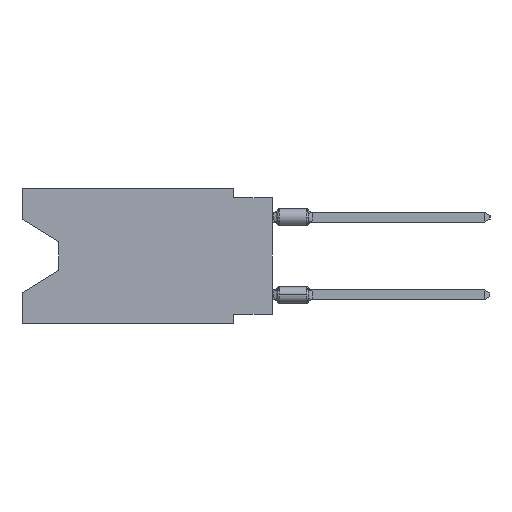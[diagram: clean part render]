
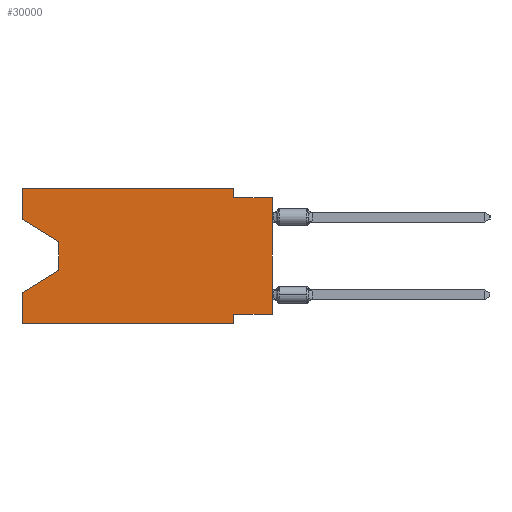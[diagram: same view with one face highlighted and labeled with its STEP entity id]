
A CAD part, left-side view. The second image highlights one B-rep face of the part: STEP entity #30000.
In plain terms, the highlighted planar face has unit normal (-1, 0, 0).
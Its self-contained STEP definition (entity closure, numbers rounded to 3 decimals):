
#176 = ORIENTED_EDGE ( 'NONE', *, *, #2564, .F. ) ;
#928 = VECTOR ( 'NONE', #32662, 1000. ) ;
#1116 = EDGE_CURVE ( 'NONE', #18634, #1347, #31646, .T. ) ;
#1347 = VERTEX_POINT ( 'NONE', #36862 ) ;
#2201 = DIRECTION ( 'NONE',  ( 0., 0., -1. ) ) ;
#2564 = EDGE_CURVE ( 'NONE', #3767, #1347, #11342, .T. ) ;
#3525 = VERTEX_POINT ( 'NONE', #20771 ) ;
#3580 = DIRECTION ( 'NONE',  ( 0., 0., 1. ) ) ;
#3767 = VERTEX_POINT ( 'NONE', #25257 ) ;
#4405 = EDGE_CURVE ( 'NONE', #15821, #12449, #11869, .T. ) ;
#4849 = CARTESIAN_POINT ( 'NONE',  ( 0., 13.97, -5.385 ) ) ;
#4953 = VECTOR ( 'NONE', #6127, 1000. ) ;
#4959 = DIRECTION ( 'NONE',  ( 0., -1., 0. ) ) ;
#5584 = CARTESIAN_POINT ( 'NONE',  ( 0., 2.54, -8.89 ) ) ;
#6069 = ORIENTED_EDGE ( 'NONE', *, *, #1116, .T. ) ;
#6127 = DIRECTION ( 'NONE',  ( 0., 1., 0. ) ) ;
#7717 = LINE ( 'NONE', #35167, #36798 ) ;
#8383 = DIRECTION ( 'NONE',  ( 0., -1., 0. ) ) ;
#9143 = CARTESIAN_POINT ( 'NONE',  ( 0., 13.97, -3.505 ) ) ;
#9159 = EDGE_CURVE ( 'NONE', #13195, #34096, #35882, .T. ) ;
#9327 = CARTESIAN_POINT ( 'NONE',  ( 0., 0., 0. ) ) ;
#9339 = VECTOR ( 'NONE', #11056, 1000. ) ;
#9959 = DIRECTION ( 'NONE',  ( 0., 0., 1. ) ) ;
#10021 = CARTESIAN_POINT ( 'NONE',  ( 0., 16.383, -6.852 ) ) ;
#10416 = EDGE_CURVE ( 'NONE', #3525, #28910, #37187, .T. ) ;
#11056 = DIRECTION ( 'NONE',  ( 0., 0., 1. ) ) ;
#11342 = LINE ( 'NONE', #23831, #928 ) ;
#11869 = LINE ( 'NONE', #18402, #35705 ) ;
#12194 = VECTOR ( 'NONE', #29258, 1000. ) ;
#12449 = VERTEX_POINT ( 'NONE', #38526 ) ;
#13195 = VERTEX_POINT ( 'NONE', #34039 ) ;
#13640 = CARTESIAN_POINT ( 'NONE',  ( 0., 2.54, -8.89 ) ) ;
#14303 = CARTESIAN_POINT ( 'NONE',  ( 0., 2.54, 0. ) ) ;
#15821 = VERTEX_POINT ( 'NONE', #17831 ) ;
#16364 = VECTOR ( 'NONE', #4959, 1000. ) ;
#16708 = LINE ( 'NONE', #13640, #29692 ) ;
#16748 = LINE ( 'NONE', #4849, #12194 ) ;
#16932 = VERTEX_POINT ( 'NONE', #36664 ) ;
#17381 = PLANE ( 'NONE',  #29134 ) ;
#17831 = CARTESIAN_POINT ( 'NONE',  ( 0., 16.383, 0. ) ) ;
#17938 = DIRECTION ( 'NONE',  ( 0., 0., -1. ) ) ;
#17967 = DIRECTION ( 'NONE',  ( 0., 0., -1. ) ) ;
#18402 = CARTESIAN_POINT ( 'NONE',  ( 0., 16.383, 0. ) ) ;
#18634 = VERTEX_POINT ( 'NONE', #29909 ) ;
#20553 = VECTOR ( 'NONE', #3580, 1000. ) ;
#20771 = CARTESIAN_POINT ( 'NONE',  ( 0., 13.97, -3.505 ) ) ;
#21028 = FACE_OUTER_BOUND ( 'NONE', #33484, .T. ) ;
#21438 = VERTEX_POINT ( 'NONE', #38200 ) ;
#21686 = LINE ( 'NONE', #34202, #4953 ) ;
#21790 = ORIENTED_EDGE ( 'NONE', *, *, #30013, .F. ) ;
#23721 = CARTESIAN_POINT ( 'NONE',  ( 0., 16.383, 0. ) ) ;
#23831 = CARTESIAN_POINT ( 'NONE',  ( 0., 0., -0.635 ) ) ;
#24373 = LINE ( 'NONE', #24591, #35591 ) ;
#24591 = CARTESIAN_POINT ( 'NONE',  ( 0., 16.383, -2.038 ) ) ;
#24756 = EDGE_CURVE ( 'NONE', #18634, #16932, #21686, .T. ) ;
#25257 = CARTESIAN_POINT ( 'NONE',  ( 0., 2.54, -0.635 ) ) ;
#26131 = DIRECTION ( 'NONE',  ( 0., 0., -1. ) ) ;
#26500 = CARTESIAN_POINT ( 'NONE',  ( 0., 13.97, -5.385 ) ) ;
#27456 = EDGE_CURVE ( 'NONE', #21438, #3525, #24373, .T. ) ;
#28910 = VERTEX_POINT ( 'NONE', #26500 ) ;
#28922 = ORIENTED_EDGE ( 'NONE', *, *, #27456, .T. ) ;
#29134 = AXIS2_PLACEMENT_3D ( 'NONE', #30265, #29885, #17967 ) ;
#29258 = DIRECTION ( 'NONE',  ( 0., 0.855, -0.519 ) ) ;
#29692 = VECTOR ( 'NONE', #26131, 1000. ) ;
#29885 = DIRECTION ( 'NONE',  ( 1., 0., 0. ) ) ;
#29909 = CARTESIAN_POINT ( 'NONE',  ( 0., 0., -8.255 ) ) ;
#30000 = ADVANCED_FACE ( 'NONE', ( #21028 ), #17381, .F. ) ;
#30013 = EDGE_CURVE ( 'NONE', #12449, #3767, #39878, .T. ) ;
#30256 = EDGE_CURVE ( 'NONE', #21438, #15821, #7717, .T. ) ;
#30265 = CARTESIAN_POINT ( 'NONE',  ( 0., 16.383, 0. ) ) ;
#31054 = ORIENTED_EDGE ( 'NONE', *, *, #10416, .T. ) ;
#31646 = LINE ( 'NONE', #9327, #20553 ) ;
#32076 = ORIENTED_EDGE ( 'NONE', *, *, #24756, .F. ) ;
#32662 = DIRECTION ( 'NONE',  ( 0., -1., 0. ) ) ;
#33484 = EDGE_LOOP ( 'NONE', ( #28922, #31054, #35264, #35123, #34402, #39205, #32076, #6069, #176, #21790, #35586, #36080 ) ) ;
#34039 = CARTESIAN_POINT ( 'NONE',  ( 0., 16.383, -8.89 ) ) ;
#34096 = VERTEX_POINT ( 'NONE', #5584 ) ;
#34202 = CARTESIAN_POINT ( 'NONE',  ( 0., 0., -8.255 ) ) ;
#34402 = ORIENTED_EDGE ( 'NONE', *, *, #9159, .T. ) ;
#35123 = ORIENTED_EDGE ( 'NONE', *, *, #38279, .F. ) ;
#35167 = CARTESIAN_POINT ( 'NONE',  ( 0., 16.383, 0. ) ) ;
#35264 = ORIENTED_EDGE ( 'NONE', *, *, #39337, .T. ) ;
#35586 = ORIENTED_EDGE ( 'NONE', *, *, #4405, .F. ) ;
#35591 = VECTOR ( 'NONE', #37068, 1000. ) ;
#35705 = VECTOR ( 'NONE', #8383, 1000. ) ;
#35882 = LINE ( 'NONE', #38536, #16364 ) ;
#35897 = EDGE_CURVE ( 'NONE', #16932, #34096, #16708, .T. ) ;
#36080 = ORIENTED_EDGE ( 'NONE', *, *, #30256, .F. ) ;
#36316 = VECTOR ( 'NONE', #2201, 1000. ) ;
#36421 = LINE ( 'NONE', #23721, #9339 ) ;
#36664 = CARTESIAN_POINT ( 'NONE',  ( 0., 2.54, -8.255 ) ) ;
#36798 = VECTOR ( 'NONE', #9959, 1000. ) ;
#36862 = CARTESIAN_POINT ( 'NONE',  ( 0., 0., -0.635 ) ) ;
#37068 = DIRECTION ( 'NONE',  ( 0., -0.855, -0.519 ) ) ;
#37079 = VECTOR ( 'NONE', #17938, 1000. ) ;
#37187 = LINE ( 'NONE', #9143, #37079 ) ;
#38129 = VERTEX_POINT ( 'NONE', #10021 ) ;
#38200 = CARTESIAN_POINT ( 'NONE',  ( 0., 16.383, -2.038 ) ) ;
#38279 = EDGE_CURVE ( 'NONE', #13195, #38129, #36421, .T. ) ;
#38526 = CARTESIAN_POINT ( 'NONE',  ( 0., 2.54, 0. ) ) ;
#38536 = CARTESIAN_POINT ( 'NONE',  ( 0., 16.383, -8.89 ) ) ;
#39205 = ORIENTED_EDGE ( 'NONE', *, *, #35897, .F. ) ;
#39337 = EDGE_CURVE ( 'NONE', #28910, #38129, #16748, .T. ) ;
#39878 = LINE ( 'NONE', #14303, #36316 ) ;
